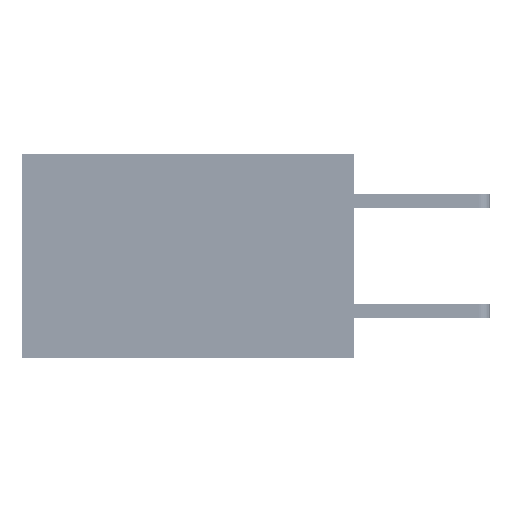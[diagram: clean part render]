
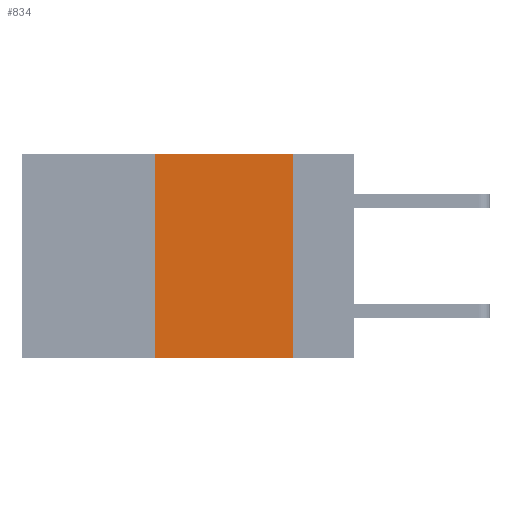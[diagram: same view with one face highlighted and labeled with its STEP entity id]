
A CAD part, left-side view. The second image highlights one B-rep face of the part: STEP entity #834.
In plain terms, the highlighted planar face has unit normal (-1, 0, 0).
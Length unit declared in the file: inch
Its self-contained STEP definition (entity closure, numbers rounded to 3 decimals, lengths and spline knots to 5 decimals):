
#834 = ADVANCED_FACE ( 'NONE', ( #36964 ), #12988, .F. ) ;
#3918 = ORIENTED_EDGE ( 'NONE', *, *, #11609, .F. ) ;
#4097 = EDGE_LOOP ( 'NONE', ( #3918, #10381, #38454, #37287 ) ) ;
#4258 = EDGE_CURVE ( 'NONE', #44536, #27496, #23599, .T. ) ;
#6309 = VECTOR ( 'NONE', #7666, 39.37008 ) ;
#7666 = DIRECTION ( 'NONE',  ( 0., 0., 1. ) ) ;
#10227 = CARTESIAN_POINT ( 'NONE',  ( 0., 0.11, 0. ) ) ;
#10381 = ORIENTED_EDGE ( 'NONE', *, *, #32302, .F. ) ;
#11166 = CARTESIAN_POINT ( 'NONE',  ( 0., 0.36, 0. ) ) ;
#11390 = CARTESIAN_POINT ( 'NONE',  ( 0., 0.36, -0.37 ) ) ;
#11434 = DIRECTION ( 'NONE',  ( 1., 0., 0. ) ) ;
#11582 = DIRECTION ( 'NONE',  ( 0., 0., -1. ) ) ;
#11609 = EDGE_CURVE ( 'NONE', #32974, #25599, #16903, .T. ) ;
#12988 = PLANE ( 'NONE',  #19861 ) ;
#13167 = CARTESIAN_POINT ( 'NONE',  ( 0., 0.11, 0. ) ) ;
#16903 = LINE ( 'NONE', #13167, #34185 ) ;
#19861 = AXIS2_PLACEMENT_3D ( 'NONE', #25019, #11434, #11582 ) ;
#20276 = CARTESIAN_POINT ( 'NONE',  ( 0., 0.6, 0. ) ) ;
#23599 = LINE ( 'NONE', #41916, #6309 ) ;
#23745 = DIRECTION ( 'NONE',  ( 0., -1., 0. ) ) ;
#24175 = DIRECTION ( 'NONE',  ( 0., 0., -1. ) ) ;
#25019 = CARTESIAN_POINT ( 'NONE',  ( 0., 0.6, 0. ) ) ;
#25117 = LINE ( 'NONE', #36499, #33248 ) ;
#25599 = VERTEX_POINT ( 'NONE', #35382 ) ;
#27496 = VERTEX_POINT ( 'NONE', #11166 ) ;
#29045 = EDGE_CURVE ( 'NONE', #44536, #25599, #25117, .T. ) ;
#32302 = EDGE_CURVE ( 'NONE', #27496, #32974, #33477, .T. ) ;
#32974 = VERTEX_POINT ( 'NONE', #10227 ) ;
#33248 = VECTOR ( 'NONE', #36819, 39.37008 ) ;
#33477 = LINE ( 'NONE', #20276, #37236 ) ;
#34185 = VECTOR ( 'NONE', #24175, 39.37008 ) ;
#35382 = CARTESIAN_POINT ( 'NONE',  ( 0., 0.11, -0.37 ) ) ;
#36499 = CARTESIAN_POINT ( 'NONE',  ( 0., 0.6, -0.37 ) ) ;
#36819 = DIRECTION ( 'NONE',  ( 0., -1., 0. ) ) ;
#36964 = FACE_OUTER_BOUND ( 'NONE', #4097, .T. ) ;
#37236 = VECTOR ( 'NONE', #23745, 39.37008 ) ;
#37287 = ORIENTED_EDGE ( 'NONE', *, *, #29045, .T. ) ;
#38454 = ORIENTED_EDGE ( 'NONE', *, *, #4258, .F. ) ;
#41916 = CARTESIAN_POINT ( 'NONE',  ( 0., 0.36, 0. ) ) ;
#44536 = VERTEX_POINT ( 'NONE', #11390 ) ;
